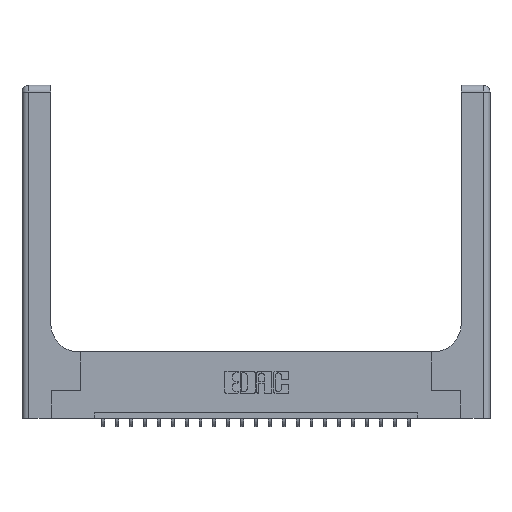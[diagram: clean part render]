
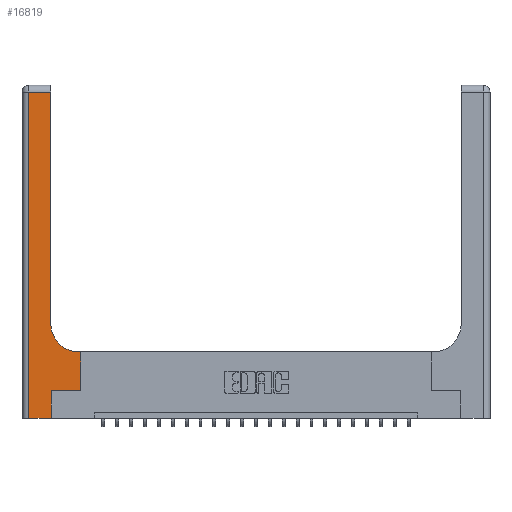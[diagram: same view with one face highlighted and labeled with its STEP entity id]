
A CAD part, top view. The second image highlights one B-rep face of the part: STEP entity #16819.
In plain terms, the highlighted planar face has unit normal (0, 0, 1).
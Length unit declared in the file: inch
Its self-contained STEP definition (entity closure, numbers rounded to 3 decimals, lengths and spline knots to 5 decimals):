
#128 = DIRECTION ( 'NONE',  ( 0., 1., 0. ) ) ;
#181 = VERTEX_POINT ( 'NONE', #14518 ) ;
#312 = ORIENTED_EDGE ( 'NONE', *, *, #7747, .T. ) ;
#499 = LINE ( 'NONE', #14929, #4633 ) ;
#848 = VERTEX_POINT ( 'NONE', #2366 ) ;
#1130 = VECTOR ( 'NONE', #5572, 39.37008 ) ;
#1290 = VECTOR ( 'NONE', #128, 39.37008 ) ;
#1363 = AXIS2_PLACEMENT_3D ( 'NONE', #20413, #10293, #22087 ) ;
#1616 = VECTOR ( 'NONE', #10327, 39.37008 ) ;
#1653 = CARTESIAN_POINT ( 'NONE',  ( 0.51, 0.6, 0.37 ) ) ;
#2249 = CARTESIAN_POINT ( 'NONE',  ( 0., 0., 0.37 ) ) ;
#2366 = CARTESIAN_POINT ( 'NONE',  ( 0.265, 0.25, 0.37 ) ) ;
#2367 = VERTEX_POINT ( 'NONE', #17188 ) ;
#2528 = ORIENTED_EDGE ( 'NONE', *, *, #6737, .T. ) ;
#2551 = EDGE_LOOP ( 'NONE', ( #4459, #312, #9522, #14028, #6049, #10605, #15631, #2528, #7093 ) ) ;
#2731 = CARTESIAN_POINT ( 'NONE',  ( 0.26, 2.94, 0.37 ) ) ;
#3619 = CARTESIAN_POINT ( 'NONE',  ( 0.26, 3., 0.37 ) ) ;
#3853 = VECTOR ( 'NONE', #14222, 39.37008 ) ;
#3869 = EDGE_CURVE ( 'NONE', #19095, #16557, #14351, .T. ) ;
#3969 = CARTESIAN_POINT ( 'NONE',  ( 0.528, 0.25, 0.37 ) ) ;
#4181 = AXIS2_PLACEMENT_3D ( 'NONE', #18596, #8499, #20342 ) ;
#4355 = LINE ( 'NONE', #7400, #9430 ) ;
#4459 = ORIENTED_EDGE ( 'NONE', *, *, #3869, .T. ) ;
#4494 = FACE_OUTER_BOUND ( 'NONE', #2551, .T. ) ;
#4633 = VECTOR ( 'NONE', #6441, 39.37008 ) ;
#4726 = CARTESIAN_POINT ( 'NONE',  ( 0.528, 0.6, 0.37 ) ) ;
#5042 = VECTOR ( 'NONE', #9838, 39.37008 ) ;
#5468 = EDGE_CURVE ( 'NONE', #9480, #19095, #19516, .T. ) ;
#5572 = DIRECTION ( 'NONE',  ( 0., 1., 0. ) ) ;
#5934 = LINE ( 'NONE', #18623, #1290 ) ;
#6049 = ORIENTED_EDGE ( 'NONE', *, *, #11489, .T. ) ;
#6359 = VECTOR ( 'NONE', #13845, 39.37008 ) ;
#6441 = DIRECTION ( 'NONE',  ( 0., -1., 0. ) ) ;
#6584 = EDGE_CURVE ( 'NONE', #12096, #2367, #499, .T. ) ;
#6737 = EDGE_CURVE ( 'NONE', #21493, #9480, #20302, .T. ) ;
#7093 = ORIENTED_EDGE ( 'NONE', *, *, #5468, .T. ) ;
#7400 = CARTESIAN_POINT ( 'NONE',  ( 0.265, 0.25, 0.37 ) ) ;
#7747 = EDGE_CURVE ( 'NONE', #16557, #12096, #10113, .T. ) ;
#8499 = DIRECTION ( 'NONE',  ( 0., 0., -1. ) ) ;
#9430 = VECTOR ( 'NONE', #14249, 39.37008 ) ;
#9480 = VERTEX_POINT ( 'NONE', #1653 ) ;
#9522 = ORIENTED_EDGE ( 'NONE', *, *, #6584, .T. ) ;
#9838 = DIRECTION ( 'NONE',  ( -1., 0., 0. ) ) ;
#10113 = LINE ( 'NONE', #18209, #5042 ) ;
#10293 = DIRECTION ( 'NONE',  ( 0., 0., -1. ) ) ;
#10327 = DIRECTION ( 'NONE',  ( -1., 0., 0. ) ) ;
#10605 = ORIENTED_EDGE ( 'NONE', *, *, #19666, .T. ) ;
#11489 = EDGE_CURVE ( 'NONE', #181, #848, #5934, .T. ) ;
#12096 = VERTEX_POINT ( 'NONE', #19990 ) ;
#13845 = DIRECTION ( 'NONE',  ( 0., 1., 0. ) ) ;
#14028 = ORIENTED_EDGE ( 'NONE', *, *, #18348, .T. ) ;
#14222 = DIRECTION ( 'NONE',  ( 1., 0., 0. ) ) ;
#14249 = DIRECTION ( 'NONE',  ( 1., 0., 0. ) ) ;
#14351 = LINE ( 'NONE', #3619, #6359 ) ;
#14518 = CARTESIAN_POINT ( 'NONE',  ( 0.265, 0., 0.37 ) ) ;
#14929 = CARTESIAN_POINT ( 'NONE',  ( 0.06, 3., 0.37 ) ) ;
#15260 = PLANE ( 'NONE',  #4181 ) ;
#15351 = LINE ( 'NONE', #15750, #1130 ) ;
#15631 = ORIENTED_EDGE ( 'NONE', *, *, #17532, .T. ) ;
#15750 = CARTESIAN_POINT ( 'NONE',  ( 0.528, 0.25, 0.37 ) ) ;
#16557 = VERTEX_POINT ( 'NONE', #2731 ) ;
#16819 = ADVANCED_FACE ( 'NONE', ( #4494 ), #15260, .F. ) ;
#16865 = LINE ( 'NONE', #2249, #3853 ) ;
#17188 = CARTESIAN_POINT ( 'NONE',  ( 0.06, 0., 0.37 ) ) ;
#17532 = EDGE_CURVE ( 'NONE', #19652, #21493, #15351, .T. ) ;
#18209 = CARTESIAN_POINT ( 'NONE',  ( 0., 2.94, 0.37 ) ) ;
#18348 = EDGE_CURVE ( 'NONE', #2367, #181, #16865, .T. ) ;
#18596 = CARTESIAN_POINT ( 'NONE',  ( 0., 3., 0.37 ) ) ;
#18623 = CARTESIAN_POINT ( 'NONE',  ( 0.265, 0., 0.37 ) ) ;
#18696 = CARTESIAN_POINT ( 'NONE',  ( 0.26, 0.6, 0.37 ) ) ;
#19095 = VERTEX_POINT ( 'NONE', #19333 ) ;
#19333 = CARTESIAN_POINT ( 'NONE',  ( 0.26, 0.85, 0.37 ) ) ;
#19516 = CIRCLE ( 'NONE', #1363, 0.25 ) ;
#19652 = VERTEX_POINT ( 'NONE', #3969 ) ;
#19666 = EDGE_CURVE ( 'NONE', #848, #19652, #4355, .T. ) ;
#19990 = CARTESIAN_POINT ( 'NONE',  ( 0.06, 2.94, 0.37 ) ) ;
#20302 = LINE ( 'NONE', #18696, #1616 ) ;
#20342 = DIRECTION ( 'NONE',  ( -1., 0., 0. ) ) ;
#20413 = CARTESIAN_POINT ( 'NONE',  ( 0.51, 0.85, 0.37 ) ) ;
#21493 = VERTEX_POINT ( 'NONE', #4726 ) ;
#22087 = DIRECTION ( 'NONE',  ( 1., 0., 0. ) ) ;
